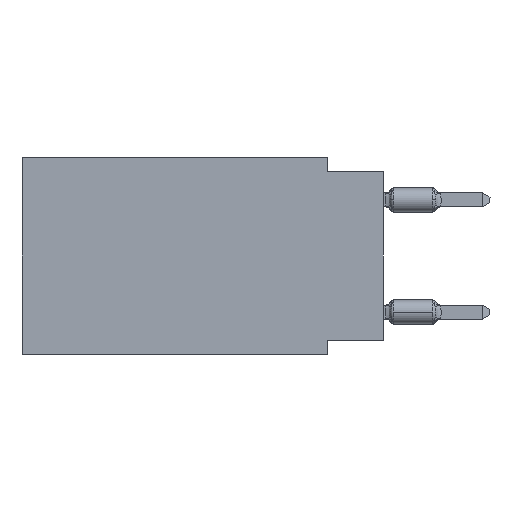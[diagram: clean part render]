
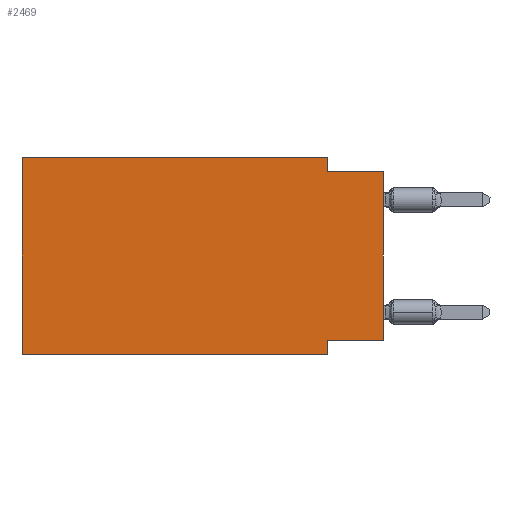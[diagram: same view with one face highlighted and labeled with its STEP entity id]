
A CAD part, left-side view. The second image highlights one B-rep face of the part: STEP entity #2469.
In plain terms, the highlighted planar face has unit normal (-1, 0, 0).
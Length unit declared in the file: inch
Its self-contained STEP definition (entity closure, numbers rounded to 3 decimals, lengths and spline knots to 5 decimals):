
#219 = ORIENTED_EDGE ( 'NONE', *, *, #26169, .F. ) ;
#1232 = ORIENTED_EDGE ( 'NONE', *, *, #16035, .F. ) ;
#1563 = PLANE ( 'NONE',  #20934 ) ;
#1976 = LINE ( 'NONE', #15683, #23921 ) ;
#1982 = CARTESIAN_POINT ( 'NONE',  ( 0., 0.1, -0.35 ) ) ;
#2469 = ADVANCED_FACE ( 'NONE', ( #20585 ), #1563, .F. ) ;
#3623 = EDGE_CURVE ( 'NONE', #7129, #4919, #26825, .T. ) ;
#3919 = ORIENTED_EDGE ( 'NONE', *, *, #10412, .T. ) ;
#4919 = VERTEX_POINT ( 'NONE', #1982 ) ;
#5043 = ORIENTED_EDGE ( 'NONE', *, *, #3623, .T. ) ;
#5563 = LINE ( 'NONE', #23266, #22198 ) ;
#5963 = DIRECTION ( 'NONE',  ( 0., 0., 1. ) ) ;
#6303 = VERTEX_POINT ( 'NONE', #18860 ) ;
#6840 = CARTESIAN_POINT ( 'NONE',  ( 0., 0., -0.025 ) ) ;
#7129 = VERTEX_POINT ( 'NONE', #16759 ) ;
#7187 = EDGE_CURVE ( 'NONE', #6303, #4919, #5563, .T. ) ;
#7820 = DIRECTION ( 'NONE',  ( 0., -1., 0. ) ) ;
#8300 = LINE ( 'NONE', #10517, #19300 ) ;
#10040 = CARTESIAN_POINT ( 'NONE',  ( 0., 0.645, -0.35 ) ) ;
#10158 = DIRECTION ( 'NONE',  ( 0., 0., -1. ) ) ;
#10373 = VERTEX_POINT ( 'NONE', #13484 ) ;
#10412 = EDGE_CURVE ( 'NONE', #15947, #15300, #18591, .T. ) ;
#10517 = CARTESIAN_POINT ( 'NONE',  ( 0., 0., -0.025 ) ) ;
#10629 = DIRECTION ( 'NONE',  ( 0., 0., -1. ) ) ;
#11255 = VECTOR ( 'NONE', #18157, 39.37008 ) ;
#11638 = CARTESIAN_POINT ( 'NONE',  ( 0., 0.1, 0. ) ) ;
#13465 = EDGE_CURVE ( 'NONE', #10373, #26541, #1976, .T. ) ;
#13484 = CARTESIAN_POINT ( 'NONE',  ( 0., 0.645, 0. ) ) ;
#13664 = ORIENTED_EDGE ( 'NONE', *, *, #21639, .F. ) ;
#14589 = LINE ( 'NONE', #26930, #26536 ) ;
#15072 = VECTOR ( 'NONE', #5963, 39.37008 ) ;
#15300 = VERTEX_POINT ( 'NONE', #6840 ) ;
#15317 = ORIENTED_EDGE ( 'NONE', *, *, #20346, .F. ) ;
#15683 = CARTESIAN_POINT ( 'NONE',  ( 0., 0.645, 0. ) ) ;
#15937 = LINE ( 'NONE', #11638, #11255 ) ;
#15947 = VERTEX_POINT ( 'NONE', #21332 ) ;
#16035 = EDGE_CURVE ( 'NONE', #26114, #15300, #8300, .T. ) ;
#16645 = LINE ( 'NONE', #24812, #20736 ) ;
#16759 = CARTESIAN_POINT ( 'NONE',  ( 0., 0.645, -0.35 ) ) ;
#16823 = ORIENTED_EDGE ( 'NONE', *, *, #13465, .F. ) ;
#18157 = DIRECTION ( 'NONE',  ( 0., 0., -1. ) ) ;
#18488 = DIRECTION ( 'NONE',  ( 0., 1., 0. ) ) ;
#18505 = CARTESIAN_POINT ( 'NONE',  ( 0., 0.645, 0. ) ) ;
#18591 = LINE ( 'NONE', #23025, #15072 ) ;
#18860 = CARTESIAN_POINT ( 'NONE',  ( 0., 0.1, -0.325 ) ) ;
#18980 = DIRECTION ( 'NONE',  ( 0., -1., 0. ) ) ;
#19269 = CARTESIAN_POINT ( 'NONE',  ( 0., 0.1, -0.025 ) ) ;
#19300 = VECTOR ( 'NONE', #18980, 39.37008 ) ;
#20346 = EDGE_CURVE ( 'NONE', #7129, #10373, #16645, .T. ) ;
#20585 = FACE_OUTER_BOUND ( 'NONE', #24082, .T. ) ;
#20736 = VECTOR ( 'NONE', #23648, 39.37008 ) ;
#20934 = AXIS2_PLACEMENT_3D ( 'NONE', #18505, #26948, #10158 ) ;
#21332 = CARTESIAN_POINT ( 'NONE',  ( 0., 0., -0.325 ) ) ;
#21547 = CARTESIAN_POINT ( 'NONE',  ( 0., 0.1, 0. ) ) ;
#21639 = EDGE_CURVE ( 'NONE', #15947, #6303, #14589, .T. ) ;
#22198 = VECTOR ( 'NONE', #10629, 39.37008 ) ;
#23025 = CARTESIAN_POINT ( 'NONE',  ( 0., 0., 0. ) ) ;
#23103 = ORIENTED_EDGE ( 'NONE', *, *, #7187, .F. ) ;
#23266 = CARTESIAN_POINT ( 'NONE',  ( 0., 0.1, -0.35 ) ) ;
#23648 = DIRECTION ( 'NONE',  ( 0., 0., 1. ) ) ;
#23921 = VECTOR ( 'NONE', #26077, 39.37008 ) ;
#24082 = EDGE_LOOP ( 'NONE', ( #3919, #1232, #219, #16823, #15317, #5043, #23103, #13664 ) ) ;
#24812 = CARTESIAN_POINT ( 'NONE',  ( 0., 0.645, 0. ) ) ;
#25325 = VECTOR ( 'NONE', #7820, 39.37008 ) ;
#26077 = DIRECTION ( 'NONE',  ( 0., -1., 0. ) ) ;
#26114 = VERTEX_POINT ( 'NONE', #19269 ) ;
#26169 = EDGE_CURVE ( 'NONE', #26541, #26114, #15937, .T. ) ;
#26536 = VECTOR ( 'NONE', #18488, 39.37008 ) ;
#26541 = VERTEX_POINT ( 'NONE', #21547 ) ;
#26825 = LINE ( 'NONE', #10040, #25325 ) ;
#26930 = CARTESIAN_POINT ( 'NONE',  ( 0., 0., -0.325 ) ) ;
#26948 = DIRECTION ( 'NONE',  ( 1., 0., 0. ) ) ;
